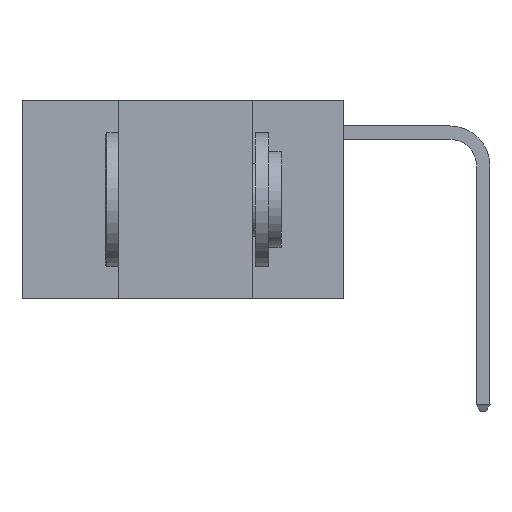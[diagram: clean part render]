
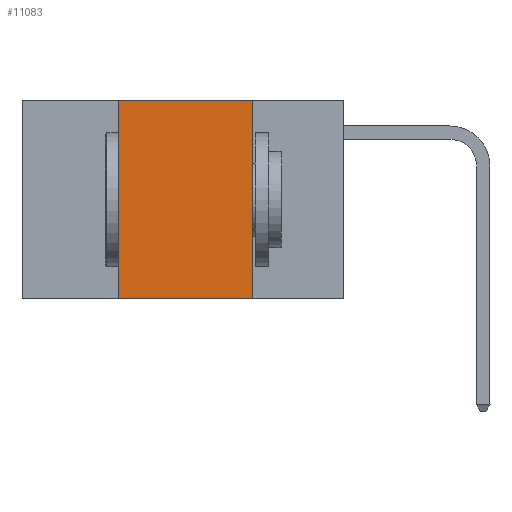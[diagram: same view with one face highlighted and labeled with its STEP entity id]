
A CAD part, left-side view. The second image highlights one B-rep face of the part: STEP entity #11083.
In plain terms, the highlighted planar face has unit normal (-1, 0, 0).
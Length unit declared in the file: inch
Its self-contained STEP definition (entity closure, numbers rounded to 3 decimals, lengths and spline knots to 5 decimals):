
#520 = DIRECTION ( 'NONE',  ( 0., 0., -1. ) ) ;
#783 = CARTESIAN_POINT ( 'NONE',  ( 0., 0.42, -0.37 ) ) ;
#961 = ORIENTED_EDGE ( 'NONE', *, *, #13938, .T. ) ;
#1105 = EDGE_LOOP ( 'NONE', ( #6148, #1703, #2833, #961 ) ) ;
#1525 = CARTESIAN_POINT ( 'NONE',  ( 0., 0.17, 0. ) ) ;
#1560 = DIRECTION ( 'NONE',  ( 0., -1., 0. ) ) ;
#1700 = VERTEX_POINT ( 'NONE', #783 ) ;
#1703 = ORIENTED_EDGE ( 'NONE', *, *, #14410, .F. ) ;
#2833 = ORIENTED_EDGE ( 'NONE', *, *, #14851, .F. ) ;
#3204 = DIRECTION ( 'NONE',  ( 1., 0., 0. ) ) ;
#4387 = DIRECTION ( 'NONE',  ( 0., 0., 1. ) ) ;
#4756 = VECTOR ( 'NONE', #4387, 39.37008 ) ;
#5217 = LINE ( 'NONE', #8561, #12529 ) ;
#6148 = ORIENTED_EDGE ( 'NONE', *, *, #17569, .F. ) ;
#6462 = VERTEX_POINT ( 'NONE', #1525 ) ;
#7051 = VERTEX_POINT ( 'NONE', #8259 ) ;
#7509 = CARTESIAN_POINT ( 'NONE',  ( 0., 0.6, -0.37 ) ) ;
#8259 = CARTESIAN_POINT ( 'NONE',  ( 0., 0.17, -0.37 ) ) ;
#8561 = CARTESIAN_POINT ( 'NONE',  ( 0., 0.6, 0. ) ) ;
#9876 = LINE ( 'NONE', #14400, #16235 ) ;
#10660 = VECTOR ( 'NONE', #15666, 39.37008 ) ;
#11083 = ADVANCED_FACE ( 'NONE', ( #12615 ), #11553, .F. ) ;
#11316 = CARTESIAN_POINT ( 'NONE',  ( 0., 0.42, 0. ) ) ;
#11553 = PLANE ( 'NONE',  #14386 ) ;
#12051 = CARTESIAN_POINT ( 'NONE',  ( 0., 0.42, 0. ) ) ;
#12529 = VECTOR ( 'NONE', #1560, 39.37008 ) ;
#12615 = FACE_OUTER_BOUND ( 'NONE', #1105, .T. ) ;
#12892 = DIRECTION ( 'NONE',  ( 0., 0., -1. ) ) ;
#13938 = EDGE_CURVE ( 'NONE', #1700, #7051, #17862, .T. ) ;
#14197 = CARTESIAN_POINT ( 'NONE',  ( 0., 0.6, 0. ) ) ;
#14386 = AXIS2_PLACEMENT_3D ( 'NONE', #14197, #3204, #12892 ) ;
#14400 = CARTESIAN_POINT ( 'NONE',  ( 0., 0.17, 0. ) ) ;
#14410 = EDGE_CURVE ( 'NONE', #15245, #6462, #5217, .T. ) ;
#14851 = EDGE_CURVE ( 'NONE', #1700, #15245, #15714, .T. ) ;
#15245 = VERTEX_POINT ( 'NONE', #12051 ) ;
#15666 = DIRECTION ( 'NONE',  ( 0., -1., 0. ) ) ;
#15714 = LINE ( 'NONE', #11316, #4756 ) ;
#16235 = VECTOR ( 'NONE', #520, 39.37008 ) ;
#17569 = EDGE_CURVE ( 'NONE', #6462, #7051, #9876, .T. ) ;
#17862 = LINE ( 'NONE', #7509, #10660 ) ;
